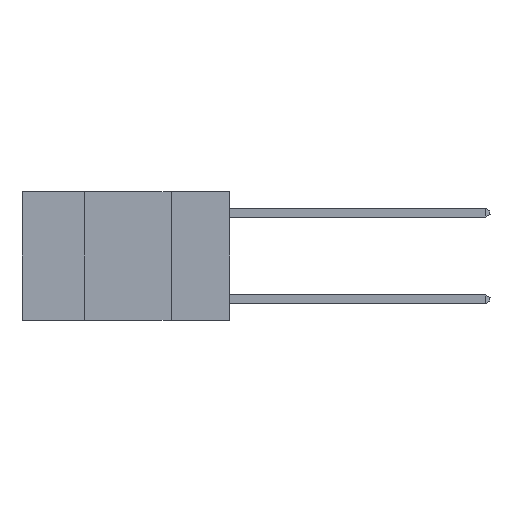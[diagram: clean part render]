
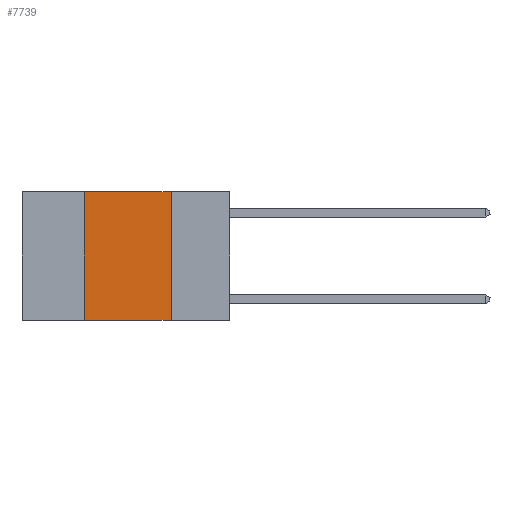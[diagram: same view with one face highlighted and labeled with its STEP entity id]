
A CAD part, left-side view. The second image highlights one B-rep face of the part: STEP entity #7739.
In plain terms, the highlighted planar face has unit normal (-1, 0, 0).
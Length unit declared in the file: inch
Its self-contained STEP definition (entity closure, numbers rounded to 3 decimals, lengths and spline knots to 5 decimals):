
#3 = VECTOR ( 'NONE', #1474, 39.37008 ) ;
#32 = LINE ( 'NONE', #4870, #10955 ) ;
#255 = VERTEX_POINT ( 'NONE', #9879 ) ;
#608 = ORIENTED_EDGE ( 'NONE', *, *, #3666, .F. ) ;
#1007 = CARTESIAN_POINT ( 'NONE',  ( 0., 0.6, 0. ) ) ;
#1311 = CARTESIAN_POINT ( 'NONE',  ( 0., 0.6, 0. ) ) ;
#1474 = DIRECTION ( 'NONE',  ( 0., -1., 0. ) ) ;
#2067 = EDGE_LOOP ( 'NONE', ( #6006, #8044, #608, #2970 ) ) ;
#2670 = LINE ( 'NONE', #6313, #3 ) ;
#2970 = ORIENTED_EDGE ( 'NONE', *, *, #6673, .T. ) ;
#3315 = CARTESIAN_POINT ( 'NONE',  ( 0., 0.42, 0. ) ) ;
#3486 = LINE ( 'NONE', #3315, #13775 ) ;
#3666 = EDGE_CURVE ( 'NONE', #7287, #9746, #3486, .T. ) ;
#3935 = DIRECTION ( 'NONE',  ( 0., 0., -1. ) ) ;
#4413 = DIRECTION ( 'NONE',  ( 0., 0., -1. ) ) ;
#4870 = CARTESIAN_POINT ( 'NONE',  ( 0., 0.17, 0. ) ) ;
#5130 = CARTESIAN_POINT ( 'NONE',  ( 0., 0.17, -0.37 ) ) ;
#6006 = ORIENTED_EDGE ( 'NONE', *, *, #11327, .F. ) ;
#6313 = CARTESIAN_POINT ( 'NONE',  ( 0., 0.6, -0.37 ) ) ;
#6673 = EDGE_CURVE ( 'NONE', #7287, #9496, #2670, .T. ) ;
#7004 = EDGE_CURVE ( 'NONE', #9746, #255, #9306, .T. ) ;
#7287 = VERTEX_POINT ( 'NONE', #12298 ) ;
#7739 = ADVANCED_FACE ( 'NONE', ( #12260 ), #12116, .F. ) ;
#8044 = ORIENTED_EDGE ( 'NONE', *, *, #7004, .F. ) ;
#8941 = CARTESIAN_POINT ( 'NONE',  ( 0., 0.42, 0. ) ) ;
#9306 = LINE ( 'NONE', #1007, #13508 ) ;
#9496 = VERTEX_POINT ( 'NONE', #5130 ) ;
#9746 = VERTEX_POINT ( 'NONE', #8941 ) ;
#9879 = CARTESIAN_POINT ( 'NONE',  ( 0., 0.17, 0. ) ) ;
#10955 = VECTOR ( 'NONE', #4413, 39.37008 ) ;
#11327 = EDGE_CURVE ( 'NONE', #255, #9496, #32, .T. ) ;
#11890 = DIRECTION ( 'NONE',  ( 0., -1., 0. ) ) ;
#12116 = PLANE ( 'NONE',  #12352 ) ;
#12196 = DIRECTION ( 'NONE',  ( 1., 0., 0. ) ) ;
#12260 = FACE_OUTER_BOUND ( 'NONE', #2067, .T. ) ;
#12298 = CARTESIAN_POINT ( 'NONE',  ( 0., 0.42, -0.37 ) ) ;
#12352 = AXIS2_PLACEMENT_3D ( 'NONE', #1311, #12196, #3935 ) ;
#12752 = DIRECTION ( 'NONE',  ( 0., 0., 1. ) ) ;
#13508 = VECTOR ( 'NONE', #11890, 39.37008 ) ;
#13775 = VECTOR ( 'NONE', #12752, 39.37008 ) ;
